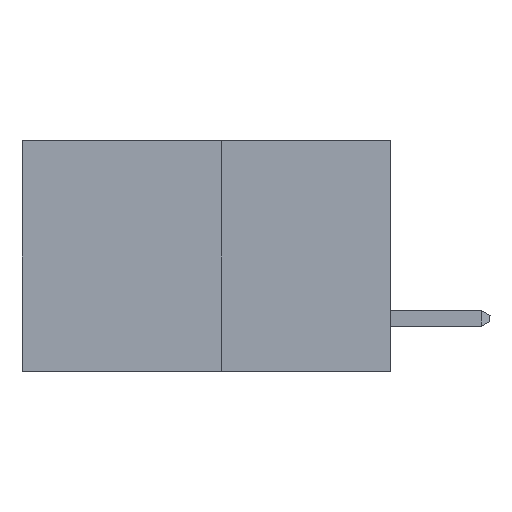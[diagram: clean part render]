
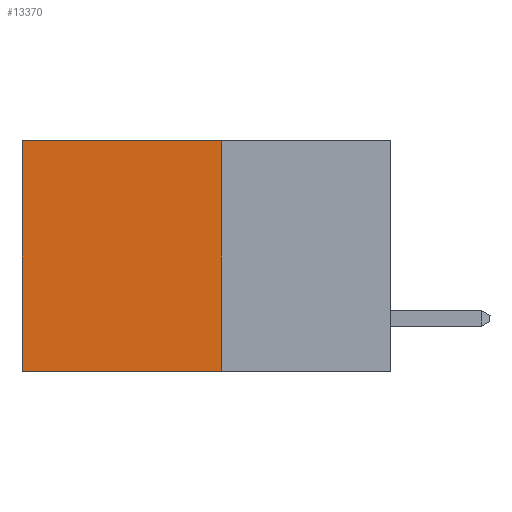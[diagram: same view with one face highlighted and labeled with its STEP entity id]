
A CAD part, left-side view. The second image highlights one B-rep face of the part: STEP entity #13370.
In plain terms, the highlighted planar face has unit normal (-1, 0, 0).
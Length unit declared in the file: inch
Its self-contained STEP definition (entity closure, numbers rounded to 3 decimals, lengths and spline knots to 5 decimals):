
#524 = VERTEX_POINT ( 'NONE', #9661 ) ;
#902 = DIRECTION ( 'NONE',  ( 0., 0., -1. ) ) ;
#997 = VERTEX_POINT ( 'NONE', #5854 ) ;
#1040 = CARTESIAN_POINT ( 'NONE',  ( 0.277, 0.27, -0.37 ) ) ;
#1109 = VECTOR ( 'NONE', #6808, 39.37008 ) ;
#1474 = LINE ( 'NONE', #1595, #1109 ) ;
#1557 = ORIENTED_EDGE ( 'NONE', *, *, #2817, .F. ) ;
#1595 = CARTESIAN_POINT ( 'NONE',  ( 0.277, 0.27, -0.37 ) ) ;
#2817 = EDGE_CURVE ( 'NONE', #997, #524, #1474, .T. ) ;
#2877 = LINE ( 'NONE', #4403, #13312 ) ;
#3069 = FACE_OUTER_BOUND ( 'NONE', #11694, .T. ) ;
#4213 = VECTOR ( 'NONE', #11464, 39.37008 ) ;
#4295 = VERTEX_POINT ( 'NONE', #7114 ) ;
#4403 = CARTESIAN_POINT ( 'NONE',  ( 0.277, 0.27, 0. ) ) ;
#4414 = DIRECTION ( 'NONE',  ( 0., 0., -1. ) ) ;
#4466 = DIRECTION ( 'NONE',  ( 0., 1., 0. ) ) ;
#4485 = EDGE_CURVE ( 'NONE', #4295, #997, #10023, .T. ) ;
#4956 = ORIENTED_EDGE ( 'NONE', *, *, #4485, .F. ) ;
#5422 = EDGE_CURVE ( 'NONE', #4295, #9855, #2877, .T. ) ;
#5854 = CARTESIAN_POINT ( 'NONE',  ( 0.277, 0.27, -0.37 ) ) ;
#6590 = ORIENTED_EDGE ( 'NONE', *, *, #5422, .T. ) ;
#6715 = ORIENTED_EDGE ( 'NONE', *, *, #8910, .T. ) ;
#6808 = DIRECTION ( 'NONE',  ( 0., 1., 0. ) ) ;
#7114 = CARTESIAN_POINT ( 'NONE',  ( 0.277, 0.27, 0. ) ) ;
#7564 = CARTESIAN_POINT ( 'NONE',  ( 0.277, 0.27, -0.37 ) ) ;
#7981 = AXIS2_PLACEMENT_3D ( 'NONE', #7564, #10521, #4414 ) ;
#8910 = EDGE_CURVE ( 'NONE', #9855, #524, #9998, .T. ) ;
#9661 = CARTESIAN_POINT ( 'NONE',  ( 0.277, 0.59, -0.37 ) ) ;
#9713 = VECTOR ( 'NONE', #902, 39.37008 ) ;
#9855 = VERTEX_POINT ( 'NONE', #12870 ) ;
#9998 = LINE ( 'NONE', #13429, #4213 ) ;
#10023 = LINE ( 'NONE', #1040, #9713 ) ;
#10482 = PLANE ( 'NONE',  #7981 ) ;
#10521 = DIRECTION ( 'NONE',  ( 1., 0., 0. ) ) ;
#11464 = DIRECTION ( 'NONE',  ( 0., 0., -1. ) ) ;
#11694 = EDGE_LOOP ( 'NONE', ( #6715, #1557, #4956, #6590 ) ) ;
#12870 = CARTESIAN_POINT ( 'NONE',  ( 0.277, 0.59, 0. ) ) ;
#13312 = VECTOR ( 'NONE', #4466, 39.37008 ) ;
#13370 = ADVANCED_FACE ( 'NONE', ( #3069 ), #10482, .F. ) ;
#13429 = CARTESIAN_POINT ( 'NONE',  ( 0.277, 0.59, -0.37 ) ) ;
